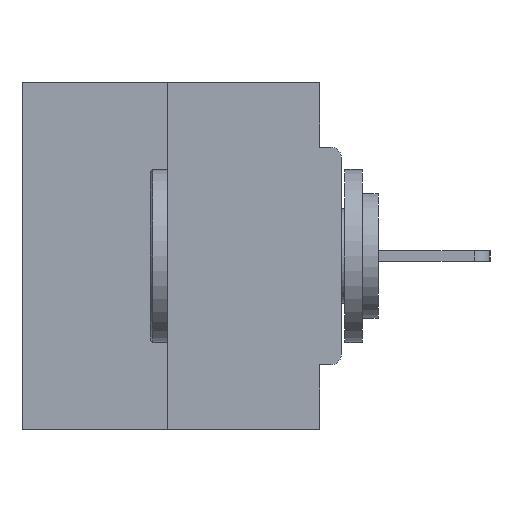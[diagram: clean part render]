
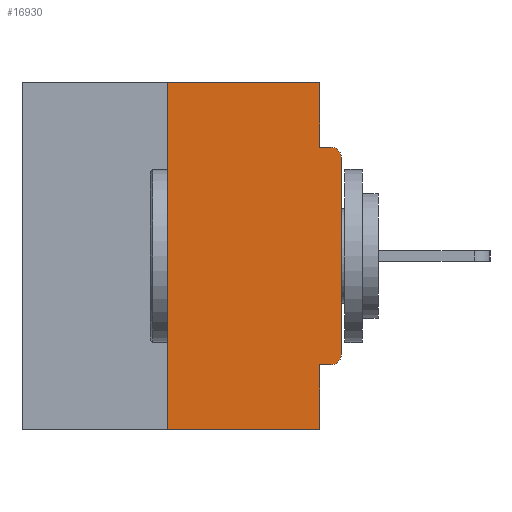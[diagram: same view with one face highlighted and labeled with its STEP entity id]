
A CAD part, left-side view. The second image highlights one B-rep face of the part: STEP entity #16930.
In plain terms, the highlighted planar face has unit normal (-1, 0, 0).
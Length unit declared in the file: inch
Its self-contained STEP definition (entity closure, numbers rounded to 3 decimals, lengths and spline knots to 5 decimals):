
#204 = AXIS2_PLACEMENT_3D ( 'NONE', #27089, #3865, #20867 ) ;
#1866 = CARTESIAN_POINT ( 'NONE',  ( 0., 0., -0.4065 ) ) ;
#2105 = DIRECTION ( 'NONE',  ( 0., -1., 0. ) ) ;
#2164 = DIRECTION ( 'NONE',  ( 0., 1., 0. ) ) ;
#2412 = VERTEX_POINT ( 'NONE', #21879 ) ;
#3021 = ORIENTED_EDGE ( 'NONE', *, *, #15188, .T. ) ;
#3131 = CARTESIAN_POINT ( 'NONE',  ( 0., 0.25, -0.5 ) ) ;
#3557 = VERTEX_POINT ( 'NONE', #11272 ) ;
#3708 = ORIENTED_EDGE ( 'NONE', *, *, #4904, .F. ) ;
#3865 = DIRECTION ( 'NONE',  ( 1., 0., 0. ) ) ;
#4042 = DIRECTION ( 'NONE',  ( 0., 0., -1. ) ) ;
#4134 = EDGE_CURVE ( 'NONE', #29634, #6457, #16901, .T. ) ;
#4240 = CARTESIAN_POINT ( 'NONE',  ( 0., 0., -0.1085 ) ) ;
#4904 = EDGE_CURVE ( 'NONE', #25256, #2412, #13608, .T. ) ;
#5081 = VERTEX_POINT ( 'NONE', #26266 ) ;
#5706 = LINE ( 'NONE', #12524, #28866 ) ;
#5735 = CARTESIAN_POINT ( 'NONE',  ( 0., 0., 0. ) ) ;
#5739 = EDGE_CURVE ( 'NONE', #25777, #20367, #6876, .T. ) ;
#6457 = VERTEX_POINT ( 'NONE', #12638 ) ;
#6876 = LINE ( 'NONE', #9362, #14139 ) ;
#7012 = ORIENTED_EDGE ( 'NONE', *, *, #25390, .T. ) ;
#7402 = CARTESIAN_POINT ( 'NONE',  ( 0., 0.031, -0.0935 ) ) ;
#7445 = VECTOR ( 'NONE', #28248, 39.37008 ) ;
#7698 = AXIS2_PLACEMENT_3D ( 'NONE', #28499, #28335, #14722 ) ;
#7766 = EDGE_CURVE ( 'NONE', #13865, #29634, #5706, .T. ) ;
#8472 = VECTOR ( 'NONE', #26967, 39.37008 ) ;
#8770 = VECTOR ( 'NONE', #4042, 39.37008 ) ;
#8792 = ORIENTED_EDGE ( 'NONE', *, *, #4134, .F. ) ;
#9147 = VECTOR ( 'NONE', #2164, 39.37008 ) ;
#9362 = CARTESIAN_POINT ( 'NONE',  ( 0., 0., -0.0935 ) ) ;
#9416 = CARTESIAN_POINT ( 'NONE',  ( 0., 0.25, 0. ) ) ;
#9806 = EDGE_CURVE ( 'NONE', #25256, #3557, #12658, .T. ) ;
#10423 = EDGE_LOOP ( 'NONE', ( #8792, #29707, #3021, #16983, #3708, #19561, #7012, #15358, #11186, #26228 ) ) ;
#10989 = EDGE_CURVE ( 'NONE', #6457, #25777, #18758, .T. ) ;
#11185 = CARTESIAN_POINT ( 'NONE',  ( 0., 0.031, 0. ) ) ;
#11186 = ORIENTED_EDGE ( 'NONE', *, *, #5739, .F. ) ;
#11272 = CARTESIAN_POINT ( 'NONE',  ( 0., 0., -0.3915 ) ) ;
#11847 = CARTESIAN_POINT ( 'NONE',  ( 0., 0.031, -0.5 ) ) ;
#12524 = CARTESIAN_POINT ( 'NONE',  ( 0., 0.25, 0. ) ) ;
#12638 = CARTESIAN_POINT ( 'NONE',  ( 0., 0.031, 0. ) ) ;
#12658 = CIRCLE ( 'NONE', #7698, 0.015 ) ;
#12844 = FACE_OUTER_BOUND ( 'NONE', #10423, .T. ) ;
#13083 = VECTOR ( 'NONE', #14590, 39.37008 ) ;
#13526 = DIRECTION ( 'NONE',  ( 0., 0., -1. ) ) ;
#13608 = LINE ( 'NONE', #1866, #9147 ) ;
#13865 = VERTEX_POINT ( 'NONE', #3131 ) ;
#14139 = VECTOR ( 'NONE', #2105, 39.37008 ) ;
#14590 = DIRECTION ( 'NONE',  ( 0., -1., 0. ) ) ;
#14631 = EDGE_CURVE ( 'NONE', #2412, #5081, #16945, .T. ) ;
#14722 = DIRECTION ( 'NONE',  ( 0., 0., -1. ) ) ;
#15120 = CIRCLE ( 'NONE', #18582, 0.015 ) ;
#15184 = DIRECTION ( 'NONE',  ( 0., 0., 1. ) ) ;
#15188 = EDGE_CURVE ( 'NONE', #13865, #5081, #15343, .T. ) ;
#15327 = LINE ( 'NONE', #5735, #19676 ) ;
#15343 = LINE ( 'NONE', #22459, #8472 ) ;
#15358 = ORIENTED_EDGE ( 'NONE', *, *, #21888, .T. ) ;
#16901 = LINE ( 'NONE', #26654, #13083 ) ;
#16930 = ADVANCED_FACE ( 'NONE', ( #12844 ), #22274, .F. ) ;
#16945 = LINE ( 'NONE', #11847, #7445 ) ;
#16983 = ORIENTED_EDGE ( 'NONE', *, *, #14631, .F. ) ;
#18582 = AXIS2_PLACEMENT_3D ( 'NONE', #25595, #28212, #13526 ) ;
#18758 = LINE ( 'NONE', #11185, #8770 ) ;
#19458 = VERTEX_POINT ( 'NONE', #4240 ) ;
#19561 = ORIENTED_EDGE ( 'NONE', *, *, #9806, .T. ) ;
#19676 = VECTOR ( 'NONE', #15184, 39.37008 ) ;
#20367 = VERTEX_POINT ( 'NONE', #30165 ) ;
#20867 = DIRECTION ( 'NONE',  ( 0., 0., -1. ) ) ;
#21879 = CARTESIAN_POINT ( 'NONE',  ( 0., 0.031, -0.4065 ) ) ;
#21888 = EDGE_CURVE ( 'NONE', #19458, #20367, #15120, .T. ) ;
#22274 = PLANE ( 'NONE',  #204 ) ;
#22459 = CARTESIAN_POINT ( 'NONE',  ( 0., 0.46, -0.5 ) ) ;
#23697 = CARTESIAN_POINT ( 'NONE',  ( 0., 0.015, -0.4065 ) ) ;
#25256 = VERTEX_POINT ( 'NONE', #23697 ) ;
#25390 = EDGE_CURVE ( 'NONE', #3557, #19458, #15327, .T. ) ;
#25595 = CARTESIAN_POINT ( 'NONE',  ( 0., 0.015, -0.1085 ) ) ;
#25777 = VERTEX_POINT ( 'NONE', #7402 ) ;
#26228 = ORIENTED_EDGE ( 'NONE', *, *, #10989, .F. ) ;
#26266 = CARTESIAN_POINT ( 'NONE',  ( 0., 0.031, -0.5 ) ) ;
#26293 = DIRECTION ( 'NONE',  ( 0., 0., 1. ) ) ;
#26654 = CARTESIAN_POINT ( 'NONE',  ( 0., 0.46, 0. ) ) ;
#26967 = DIRECTION ( 'NONE',  ( 0., -1., 0. ) ) ;
#27089 = CARTESIAN_POINT ( 'NONE',  ( 0., 0.46, 0. ) ) ;
#28212 = DIRECTION ( 'NONE',  ( -1., 0., 0. ) ) ;
#28248 = DIRECTION ( 'NONE',  ( 0., 0., -1. ) ) ;
#28335 = DIRECTION ( 'NONE',  ( -1., 0., 0. ) ) ;
#28499 = CARTESIAN_POINT ( 'NONE',  ( 0., 0.015, -0.3915 ) ) ;
#28866 = VECTOR ( 'NONE', #26293, 39.37008 ) ;
#29634 = VERTEX_POINT ( 'NONE', #9416 ) ;
#29707 = ORIENTED_EDGE ( 'NONE', *, *, #7766, .F. ) ;
#30165 = CARTESIAN_POINT ( 'NONE',  ( 0., 0.015, -0.0935 ) ) ;
